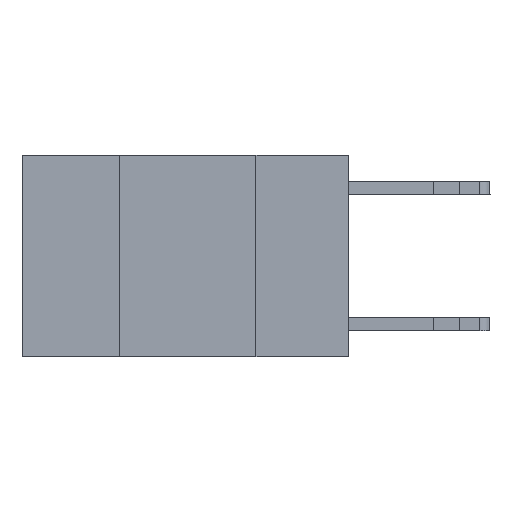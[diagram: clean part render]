
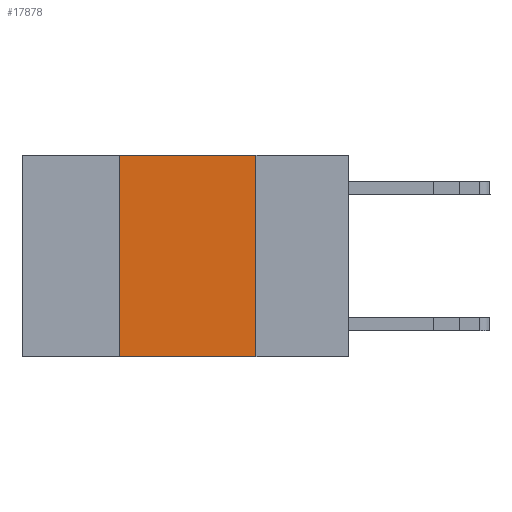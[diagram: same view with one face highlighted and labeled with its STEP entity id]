
A CAD part, left-side view. The second image highlights one B-rep face of the part: STEP entity #17878.
In plain terms, the highlighted planar face has unit normal (-1, 0, 0).
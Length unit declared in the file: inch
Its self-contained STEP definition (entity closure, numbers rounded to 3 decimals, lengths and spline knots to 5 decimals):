
#624 = LINE ( 'NONE', #12101, #15294 ) ;
#821 = DIRECTION ( 'NONE',  ( 0., -1., 0. ) ) ;
#1889 = DIRECTION ( 'NONE',  ( 0., 0., 1. ) ) ;
#2199 = DIRECTION ( 'NONE',  ( 0., -1., 0. ) ) ;
#2279 = ORIENTED_EDGE ( 'NONE', *, *, #16597, .F. ) ;
#2772 = LINE ( 'NONE', #8944, #6535 ) ;
#2916 = EDGE_CURVE ( 'NONE', #11648, #16750, #624, .T. ) ;
#2924 = EDGE_CURVE ( 'NONE', #4361, #4940, #11480, .T. ) ;
#3716 = LINE ( 'NONE', #13781, #18262 ) ;
#4361 = VERTEX_POINT ( 'NONE', #15182 ) ;
#4940 = VERTEX_POINT ( 'NONE', #18109 ) ;
#6495 = ORIENTED_EDGE ( 'NONE', *, *, #2916, .T. ) ;
#6535 = VECTOR ( 'NONE', #1889, 39.37008 ) ;
#7485 = FACE_OUTER_BOUND ( 'NONE', #9439, .T. ) ;
#7486 = CARTESIAN_POINT ( 'NONE',  ( 0., 0.42, -0.37 ) ) ;
#7754 = VECTOR ( 'NONE', #821, 39.37008 ) ;
#7766 = DIRECTION ( 'NONE',  ( 1., 0., 0. ) ) ;
#8031 = EDGE_CURVE ( 'NONE', #4940, #16750, #3716, .T. ) ;
#8944 = CARTESIAN_POINT ( 'NONE',  ( 0., 0.42, 0. ) ) ;
#9439 = EDGE_LOOP ( 'NONE', ( #16433, #13149, #2279, #6495 ) ) ;
#10940 = DIRECTION ( 'NONE',  ( 0., 0., -1. ) ) ;
#11480 = LINE ( 'NONE', #17746, #7754 ) ;
#11648 = VERTEX_POINT ( 'NONE', #7486 ) ;
#12101 = CARTESIAN_POINT ( 'NONE',  ( 0., 0.6, -0.37 ) ) ;
#12309 = CARTESIAN_POINT ( 'NONE',  ( 0., 0.17, -0.37 ) ) ;
#13149 = ORIENTED_EDGE ( 'NONE', *, *, #2924, .F. ) ;
#13781 = CARTESIAN_POINT ( 'NONE',  ( 0., 0.17, 0. ) ) ;
#15182 = CARTESIAN_POINT ( 'NONE',  ( 0., 0.42, 0. ) ) ;
#15294 = VECTOR ( 'NONE', #2199, 39.37008 ) ;
#16203 = CARTESIAN_POINT ( 'NONE',  ( 0., 0.6, 0. ) ) ;
#16433 = ORIENTED_EDGE ( 'NONE', *, *, #8031, .F. ) ;
#16597 = EDGE_CURVE ( 'NONE', #11648, #4361, #2772, .T. ) ;
#16750 = VERTEX_POINT ( 'NONE', #12309 ) ;
#17445 = AXIS2_PLACEMENT_3D ( 'NONE', #16203, #7766, #17602 ) ;
#17543 = PLANE ( 'NONE',  #17445 ) ;
#17602 = DIRECTION ( 'NONE',  ( 0., 0., -1. ) ) ;
#17746 = CARTESIAN_POINT ( 'NONE',  ( 0., 0.6, 0. ) ) ;
#17878 = ADVANCED_FACE ( 'NONE', ( #7485 ), #17543, .F. ) ;
#18109 = CARTESIAN_POINT ( 'NONE',  ( 0., 0.17, 0. ) ) ;
#18262 = VECTOR ( 'NONE', #10940, 39.37008 ) ;
